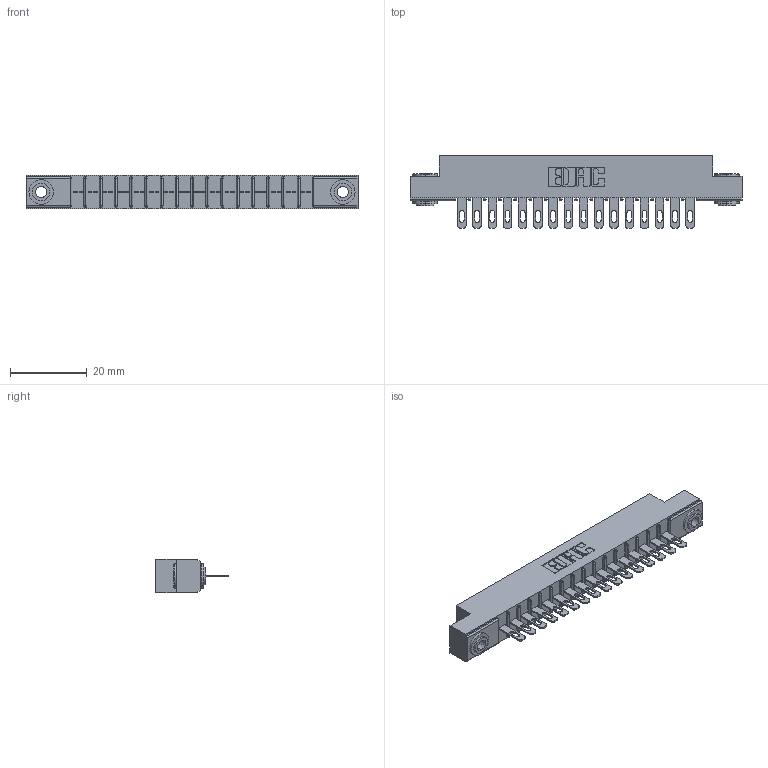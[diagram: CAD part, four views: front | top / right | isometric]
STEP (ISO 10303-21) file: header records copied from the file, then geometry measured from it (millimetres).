
FILE_DESCRIPTION (( 'STEP AP203' ), '1' );
FILE_NAME ('316-016-500-103.STEP', '2018-07-31T00:55:34', ( '' ), ( '' ), 'SwSTEP 2.0', 'SolidWorks 2016', '' );
FILE_SCHEMA (( 'CONFIG_CONTROL_DESIGN' ));
Length unit declared in the file: inch
Products named in the file (4): 306 Part_.156 Dia; 306-290-001_100; 345-250-002_345-250-002-102; 316-016-500-103
Assembly tree (19 placements, depth 2):
  316-016-500-103
    306 Part_.156 Dia
    306-290-001_100  x16
    345-250-002_345-250-002-102  x2
Bounding box: 86.41 x 18.87 x 8.71 mm (x, y, z)
Volume: 5940.1 mm3; surface area: 9091.3 mm2
Topology: 19 solids, 19 shells, 1384 faces, 3868 edges, 2488 vertices
Faces by surface type: plane 892, cylinder 420, sphere 64, cone 8
Entity records: 19518 total; most frequent: CARTESIAN_POINT 3252, DIRECTION 3224, ORIENTED_EDGE 3212, EDGE_CURVE 1606, LINE 1232, VECTOR 1232, VERTEX_POINT 1024, AXIS2_PLACEMENT_3D 996
